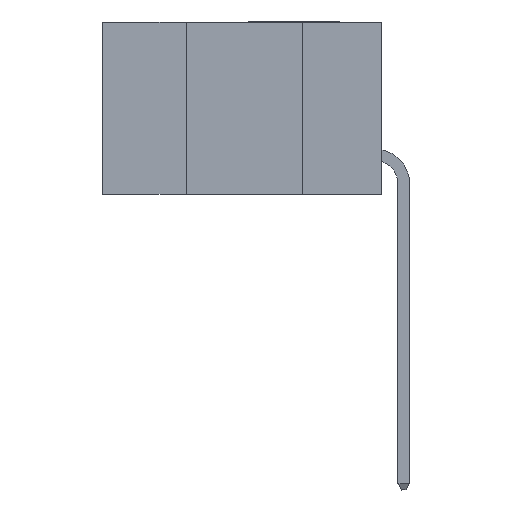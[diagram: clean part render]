
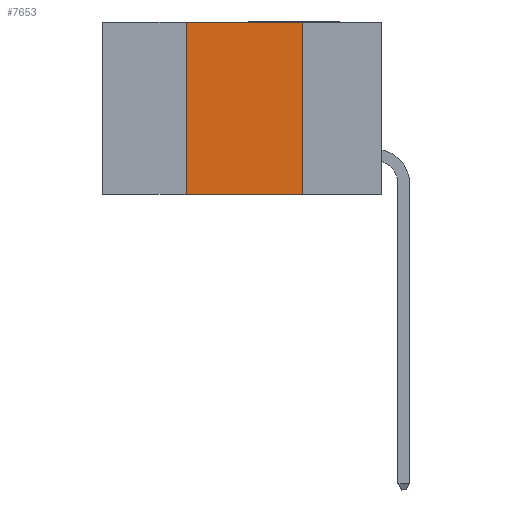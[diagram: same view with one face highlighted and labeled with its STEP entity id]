
A CAD part, left-side view. The second image highlights one B-rep face of the part: STEP entity #7653.
In plain terms, the highlighted planar face has unit normal (-1, 0, 0).
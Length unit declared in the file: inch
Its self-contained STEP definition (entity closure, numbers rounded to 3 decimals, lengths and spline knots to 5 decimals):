
#166 = DIRECTION ( 'NONE',  ( 0., 0., -1. ) ) ;
#219 = CARTESIAN_POINT ( 'NONE',  ( 0., 0.42, -0.37 ) ) ;
#273 = EDGE_CURVE ( 'NONE', #1948, #6989, #8095, .T. ) ;
#1117 = ORIENTED_EDGE ( 'NONE', *, *, #3499, .F. ) ;
#1402 = ORIENTED_EDGE ( 'NONE', *, *, #6437, .F. ) ;
#1948 = VERTEX_POINT ( 'NONE', #219 ) ;
#2281 = DIRECTION ( 'NONE',  ( 1., 0., 0. ) ) ;
#2828 = VERTEX_POINT ( 'NONE', #3025 ) ;
#2931 = LINE ( 'NONE', #7771, #6306 ) ;
#3025 = CARTESIAN_POINT ( 'NONE',  ( 0., 0.17, 0. ) ) ;
#3499 = EDGE_CURVE ( 'NONE', #5984, #2828, #8612, .T. ) ;
#3720 = ORIENTED_EDGE ( 'NONE', *, *, #273, .T. ) ;
#3864 = FACE_OUTER_BOUND ( 'NONE', #6787, .T. ) ;
#3929 = VECTOR ( 'NONE', #6706, 39.37008 ) ;
#4127 = CARTESIAN_POINT ( 'NONE',  ( 0., 0.42, 0. ) ) ;
#4375 = CARTESIAN_POINT ( 'NONE',  ( 0., 0.6, 0. ) ) ;
#4439 = DIRECTION ( 'NONE',  ( 0., 0., -1. ) ) ;
#5108 = EDGE_CURVE ( 'NONE', #2828, #6989, #2931, .T. ) ;
#5110 = ORIENTED_EDGE ( 'NONE', *, *, #5108, .F. ) ;
#5193 = AXIS2_PLACEMENT_3D ( 'NONE', #4375, #2281, #4439 ) ;
#5641 = VECTOR ( 'NONE', #6261, 39.37008 ) ;
#5984 = VERTEX_POINT ( 'NONE', #8499 ) ;
#6261 = DIRECTION ( 'NONE',  ( 0., 0., 1. ) ) ;
#6306 = VECTOR ( 'NONE', #166, 39.37008 ) ;
#6437 = EDGE_CURVE ( 'NONE', #1948, #5984, #8030, .T. ) ;
#6706 = DIRECTION ( 'NONE',  ( 0., -1., 0. ) ) ;
#6787 = EDGE_LOOP ( 'NONE', ( #5110, #1117, #1402, #3720 ) ) ;
#6898 = VECTOR ( 'NONE', #7812, 39.37008 ) ;
#6989 = VERTEX_POINT ( 'NONE', #8288 ) ;
#7152 = CARTESIAN_POINT ( 'NONE',  ( 0., 0.6, -0.37 ) ) ;
#7188 = PLANE ( 'NONE',  #5193 ) ;
#7653 = ADVANCED_FACE ( 'NONE', ( #3864 ), #7188, .F. ) ;
#7771 = CARTESIAN_POINT ( 'NONE',  ( 0., 0.17, 0. ) ) ;
#7812 = DIRECTION ( 'NONE',  ( 0., -1., 0. ) ) ;
#8030 = LINE ( 'NONE', #4127, #5641 ) ;
#8095 = LINE ( 'NONE', #7152, #6898 ) ;
#8288 = CARTESIAN_POINT ( 'NONE',  ( 0., 0.17, -0.37 ) ) ;
#8499 = CARTESIAN_POINT ( 'NONE',  ( 0., 0.42, 0. ) ) ;
#8611 = CARTESIAN_POINT ( 'NONE',  ( 0., 0.6, 0. ) ) ;
#8612 = LINE ( 'NONE', #8611, #3929 ) ;
